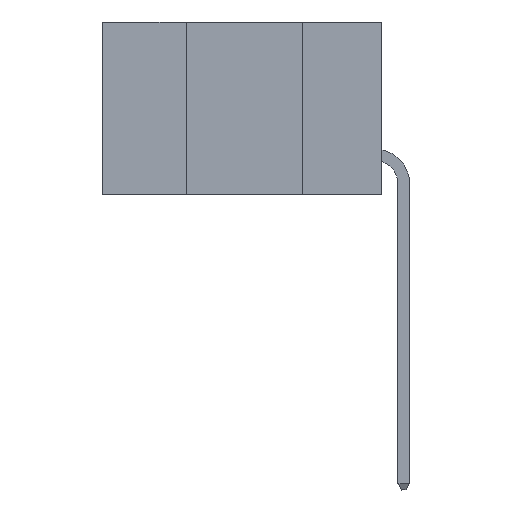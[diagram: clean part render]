
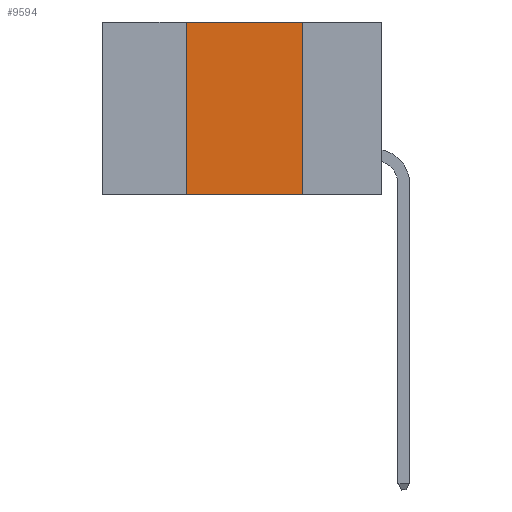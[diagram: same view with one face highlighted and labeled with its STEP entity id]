
A CAD part, left-side view. The second image highlights one B-rep face of the part: STEP entity #9594.
In plain terms, the highlighted planar face has unit normal (-1, 0, 0).
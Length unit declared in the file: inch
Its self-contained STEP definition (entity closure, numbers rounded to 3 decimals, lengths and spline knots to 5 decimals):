
#2033 = CARTESIAN_POINT ( 'NONE',  ( 0., 0.17, 0. ) ) ;
#2866 = CARTESIAN_POINT ( 'NONE',  ( 0., 0.42, 0. ) ) ;
#3385 = VECTOR ( 'NONE', #5081, 39.37008 ) ;
#5081 = DIRECTION ( 'NONE',  ( 0., 0., 1. ) ) ;
#6212 = ORIENTED_EDGE ( 'NONE', *, *, #26757, .F. ) ;
#8432 = CARTESIAN_POINT ( 'NONE',  ( 0., 0.42, -0.37 ) ) ;
#9594 = ADVANCED_FACE ( 'NONE', ( #34594 ), #24718, .F. ) ;
#9944 = VECTOR ( 'NONE', #28198, 39.37008 ) ;
#10291 = VERTEX_POINT ( 'NONE', #2866 ) ;
#12413 = VERTEX_POINT ( 'NONE', #49064 ) ;
#13133 = ORIENTED_EDGE ( 'NONE', *, *, #17525, .F. ) ;
#13461 = DIRECTION ( 'NONE',  ( 0., 0., -1. ) ) ;
#15787 = CARTESIAN_POINT ( 'NONE',  ( 0., 0.6, -0.37 ) ) ;
#16462 = CARTESIAN_POINT ( 'NONE',  ( 0., 0.42, 0. ) ) ;
#17033 = VERTEX_POINT ( 'NONE', #39579 ) ;
#17039 = ORIENTED_EDGE ( 'NONE', *, *, #18527, .T. ) ;
#17525 = EDGE_CURVE ( 'NONE', #29085, #10291, #42370, .T. ) ;
#18527 = EDGE_CURVE ( 'NONE', #29085, #17033, #20645, .T. ) ;
#18621 = EDGE_LOOP ( 'NONE', ( #6212, #41979, #13133, #17039 ) ) ;
#18715 = AXIS2_PLACEMENT_3D ( 'NONE', #44021, #36477, #13461 ) ;
#20134 = LINE ( 'NONE', #31865, #9944 ) ;
#20645 = LINE ( 'NONE', #15787, #48881 ) ;
#23852 = DIRECTION ( 'NONE',  ( 0., -1., 0. ) ) ;
#24718 = PLANE ( 'NONE',  #18715 ) ;
#26757 = EDGE_CURVE ( 'NONE', #12413, #17033, #44234, .T. ) ;
#27316 = EDGE_CURVE ( 'NONE', #10291, #12413, #20134, .T. ) ;
#28198 = DIRECTION ( 'NONE',  ( 0., -1., 0. ) ) ;
#29085 = VERTEX_POINT ( 'NONE', #8432 ) ;
#31865 = CARTESIAN_POINT ( 'NONE',  ( 0., 0.6, 0. ) ) ;
#34594 = FACE_OUTER_BOUND ( 'NONE', #18621, .T. ) ;
#36477 = DIRECTION ( 'NONE',  ( 1., 0., 0. ) ) ;
#39579 = CARTESIAN_POINT ( 'NONE',  ( 0., 0.17, -0.37 ) ) ;
#40452 = DIRECTION ( 'NONE',  ( 0., 0., -1. ) ) ;
#41979 = ORIENTED_EDGE ( 'NONE', *, *, #27316, .F. ) ;
#42370 = LINE ( 'NONE', #16462, #3385 ) ;
#44021 = CARTESIAN_POINT ( 'NONE',  ( 0., 0.6, 0. ) ) ;
#44234 = LINE ( 'NONE', #2033, #48425 ) ;
#48425 = VECTOR ( 'NONE', #40452, 39.37008 ) ;
#48881 = VECTOR ( 'NONE', #23852, 39.37008 ) ;
#49064 = CARTESIAN_POINT ( 'NONE',  ( 0., 0.17, 0. ) ) ;
